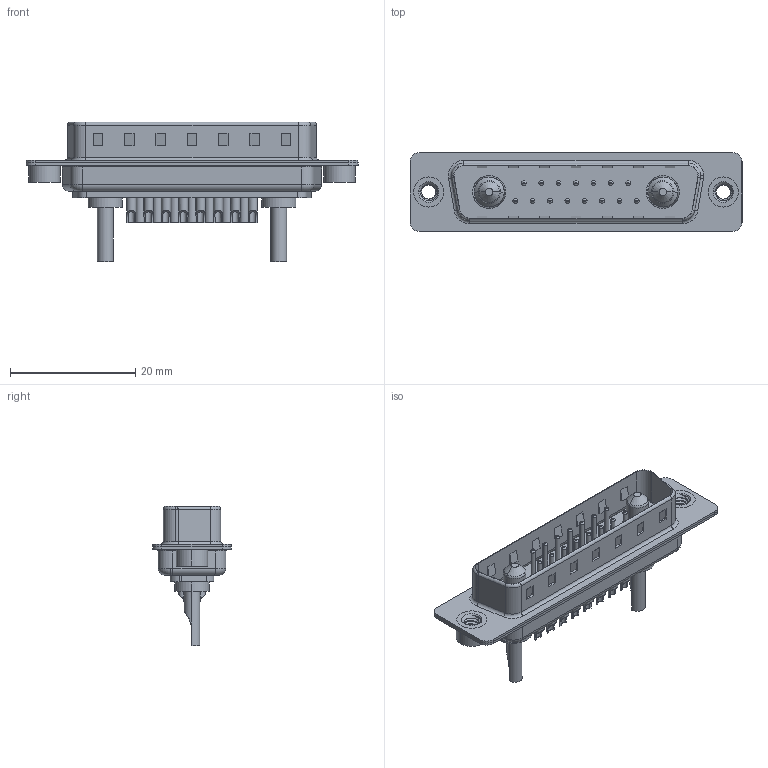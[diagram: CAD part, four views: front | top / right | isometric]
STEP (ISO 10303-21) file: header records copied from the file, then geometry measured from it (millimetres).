
FILE_DESCRIPTION (( 'STEP AP203' ), '1' );
FILE_NAME ('627-17W2622-1T2.STEP', '2019-05-27T21:51:43', ( '' ), ( '' ), 'SwSTEP 2.0', 'SolidWorks 2016', '' );
FILE_SCHEMA (( 'CONFIG_CONTROL_DESIGN' ));
Length unit declared in the file: millimetre
Products named in the file (8): 627Combo Contact Row 2_22; 627-17W2622-1T2; 627Combo Threaded Rivet_2; 627Combo Contact Row 1_22; 627Combo Shell Rear_25 Contacts; 627Combo Shell Front_25 Contacts; Power Pin_10A SC; 627Combo Housing_17W2
Assembly tree (22 placements, depth 2):
  627-17W2622-1T2
    627Combo Housing_17W2
    627Combo Shell Rear_25 Contacts
    627Combo Shell Front_25 Contacts
    627Combo Threaded Rivet_2  x2
    Power Pin_10A SC  x2
    627Combo Contact Row 1_22  x7
    627Combo Contact Row 2_22  x8
Bounding box: 53 x 12.6 x 22.3 mm (x, y, z)
Volume: 2874 mm3; surface area: 7003.2 mm2
Topology: 24 solids, 24 shells, 1021 faces, 2415 edges, 1485 vertices
Faces by surface type: cylinder 421, plane 330, torus 204, cone 56, bspline 10
Entity records: 19718 total; most frequent: CARTESIAN_POINT 4566, DIRECTION 3085, ORIENTED_EDGE 2762, EDGE_CURVE 1381, AXIS2_PLACEMENT_3D 1186, VERTEX_POINT 875, LINE 713, VECTOR 713
